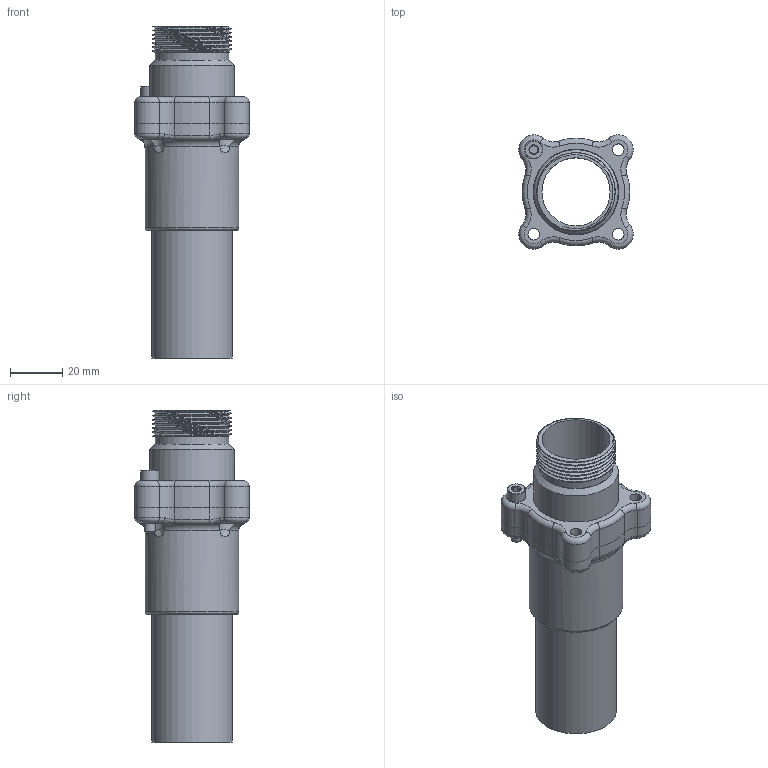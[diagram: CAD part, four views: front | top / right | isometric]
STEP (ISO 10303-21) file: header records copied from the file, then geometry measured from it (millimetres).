
FILE_DESCRIPTION(/* description */ (''),/* implementation_level */ '2;1');
FILE_NAME(/* name */ 'Adapter Assembly.step',/* time_stamp */ '2023-02-02T21:16:09-05:00',/* author */ (''),/* organization */ (''),/* preprocessor_version */ 'ST-DEVELOPER v19.2',/* originating_system */ 'Autodesk Translation Framework v11.17.0.187',/* authorisation */ '');
FILE_SCHEMA (('AUTOMOTIVE_DESIGN { 1 0 10303 214 3 1 1 }'));
Length unit declared in the file: millimetre
Products named in the file (6): 5D Tactical 1-1/4in Hose Adapter; 5D Tactical Buffer Tube Mount; Vaccum Tube 1-1/4 in.; 91290A168_NO THREADS_Alloy Steel Socket Head Screw; 5D Clamp; Hose Clamp
Assembly tree (5 placements, depth 2):
  5D Tactical 1-1/4in Hose Adapter
    5D Tactical Buffer Tube Mount
    Vaccum Tube 1-1/4 in.
    91290A168_NO THREADS_Alloy Steel Socket Head Screw
    5D Clamp
    Hose Clamp
Bounding box: 43.89 x 43.89 x 127.4 mm (x, y, z)
Volume: 45423.2 mm3; surface area: 40891.9 mm2
Topology: 5 solids, 5 shells, 157 faces, 399 edges, 256 vertices
Faces by surface type: cylinder 73, torus 38, plane 26, bspline 14, cone 6
Full cylindrical faces by diameter (mm): 4 x1, 4.5 x8, 7 x1, 7.1 x2, 26.15 x1, 27.4 x1, 28.15 x1, 28.27 x5, 30.043 x6, 31 x2, 32.4 x1, 32.9 x1, 34.3 x1, 34.6 x1, 36 x1
Entity records: 7886 total; most frequent: CARTESIAN_POINT 3907, DIRECTION 807, ORIENTED_EDGE 798, EDGE_CURVE 399, AXIS2_PLACEMENT_3D 361, VERTEX_POINT 256, CIRCLE 207, EDGE_LOOP 189
